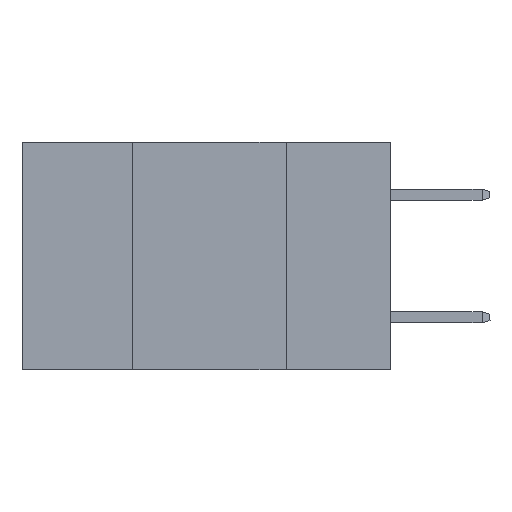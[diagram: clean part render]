
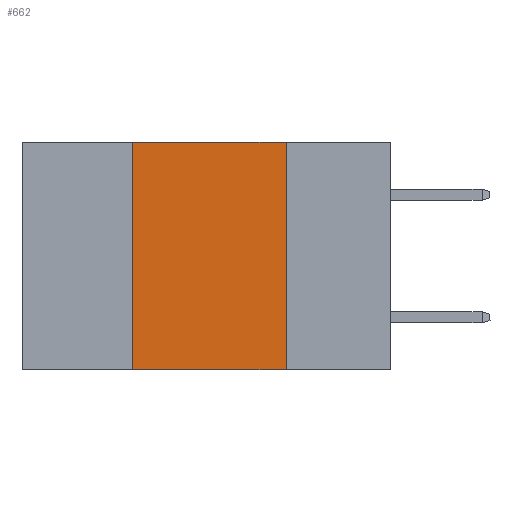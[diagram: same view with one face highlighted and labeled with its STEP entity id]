
A CAD part, left-side view. The second image highlights one B-rep face of the part: STEP entity #662.
In plain terms, the highlighted planar face has unit normal (-1, 0, 0).
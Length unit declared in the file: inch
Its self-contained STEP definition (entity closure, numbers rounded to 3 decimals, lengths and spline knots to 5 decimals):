
#662 = ADVANCED_FACE ( 'NONE', ( #744 ), #15277, .F. ) ;
#744 = FACE_OUTER_BOUND ( 'NONE', #10291, .T. ) ;
#1401 = CARTESIAN_POINT ( 'NONE',  ( 0., 0.42, -0.37 ) ) ;
#1527 = VECTOR ( 'NONE', #2261, 39.37008 ) ;
#2114 = VERTEX_POINT ( 'NONE', #18348 ) ;
#2261 = DIRECTION ( 'NONE',  ( 0., -1., 0. ) ) ;
#2825 = LINE ( 'NONE', #15786, #6451 ) ;
#3715 = AXIS2_PLACEMENT_3D ( 'NONE', #15255, #15221, #15166 ) ;
#4574 = ORIENTED_EDGE ( 'NONE', *, *, #18805, .F. ) ;
#4688 = VERTEX_POINT ( 'NONE', #1401 ) ;
#4748 = VECTOR ( 'NONE', #14825, 39.37008 ) ;
#5573 = ORIENTED_EDGE ( 'NONE', *, *, #15461, .F. ) ;
#6451 = VECTOR ( 'NONE', #11512, 39.37008 ) ;
#9720 = VERTEX_POINT ( 'NONE', #14919 ) ;
#10291 = EDGE_LOOP ( 'NONE', ( #16005, #4574, #5573, #17347 ) ) ;
#10571 = CARTESIAN_POINT ( 'NONE',  ( 0., 0.42, 0. ) ) ;
#11410 = CARTESIAN_POINT ( 'NONE',  ( 0., 0.6, -0.37 ) ) ;
#11512 = DIRECTION ( 'NONE',  ( 0., -1., 0. ) ) ;
#12465 = CARTESIAN_POINT ( 'NONE',  ( 0., 0.42, 0. ) ) ;
#12580 = EDGE_CURVE ( 'NONE', #4688, #2114, #13207, .T. ) ;
#13207 = LINE ( 'NONE', #11410, #1527 ) ;
#13404 = CARTESIAN_POINT ( 'NONE',  ( 0., 0.17, 0. ) ) ;
#13928 = DIRECTION ( 'NONE',  ( 0., 0., 1. ) ) ;
#14825 = DIRECTION ( 'NONE',  ( 0., 0., -1. ) ) ;
#14919 = CARTESIAN_POINT ( 'NONE',  ( 0., 0.17, 0. ) ) ;
#15166 = DIRECTION ( 'NONE',  ( 0., 0., -1. ) ) ;
#15221 = DIRECTION ( 'NONE',  ( 1., 0., 0. ) ) ;
#15228 = VERTEX_POINT ( 'NONE', #10571 ) ;
#15255 = CARTESIAN_POINT ( 'NONE',  ( 0., 0.6, 0. ) ) ;
#15277 = PLANE ( 'NONE',  #3715 ) ;
#15317 = VECTOR ( 'NONE', #13928, 39.37008 ) ;
#15461 = EDGE_CURVE ( 'NONE', #4688, #15228, #15774, .T. ) ;
#15774 = LINE ( 'NONE', #12465, #15317 ) ;
#15786 = CARTESIAN_POINT ( 'NONE',  ( 0., 0.6, 0. ) ) ;
#16005 = ORIENTED_EDGE ( 'NONE', *, *, #17390, .F. ) ;
#16604 = LINE ( 'NONE', #13404, #4748 ) ;
#17347 = ORIENTED_EDGE ( 'NONE', *, *, #12580, .T. ) ;
#17390 = EDGE_CURVE ( 'NONE', #9720, #2114, #16604, .T. ) ;
#18348 = CARTESIAN_POINT ( 'NONE',  ( 0., 0.17, -0.37 ) ) ;
#18805 = EDGE_CURVE ( 'NONE', #15228, #9720, #2825, .T. ) ;
